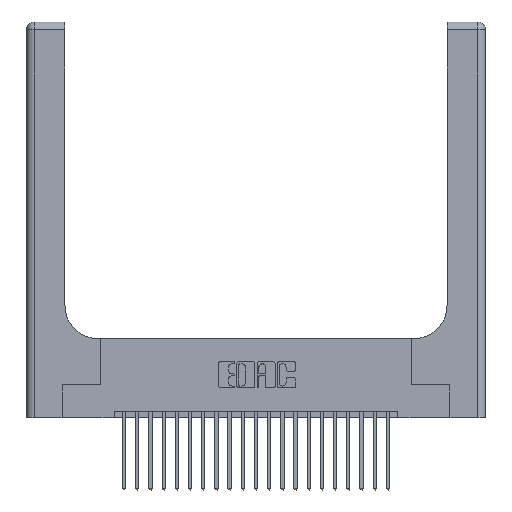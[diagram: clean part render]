
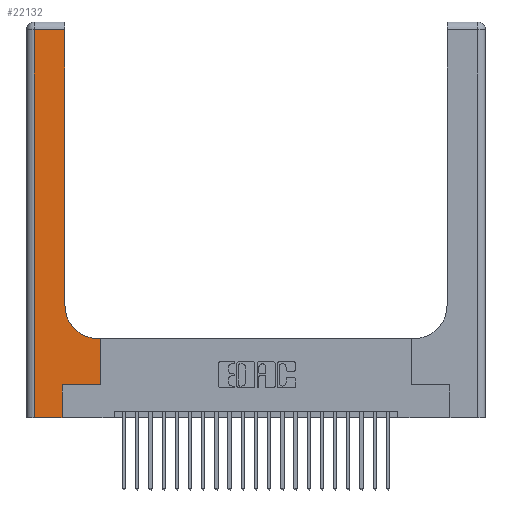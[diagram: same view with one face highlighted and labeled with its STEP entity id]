
A CAD part, top view. The second image highlights one B-rep face of the part: STEP entity #22132.
In plain terms, the highlighted planar face has unit normal (0, 0, 1).
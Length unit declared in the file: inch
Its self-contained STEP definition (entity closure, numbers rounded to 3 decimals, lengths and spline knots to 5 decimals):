
#15 = ORIENTED_EDGE ( 'NONE', *, *, #10885, .T. ) ;
#151 = VECTOR ( 'NONE', #19721, 39.37008 ) ;
#191 = VERTEX_POINT ( 'NONE', #14990 ) ;
#304 = ORIENTED_EDGE ( 'NONE', *, *, #4779, .T. ) ;
#628 = EDGE_CURVE ( 'NONE', #14026, #11535, #16744, .T. ) ;
#1269 = LINE ( 'NONE', #4823, #3941 ) ;
#1821 = ORIENTED_EDGE ( 'NONE', *, *, #12774, .T. ) ;
#1861 = LINE ( 'NONE', #20226, #16355 ) ;
#2771 = VERTEX_POINT ( 'NONE', #4696 ) ;
#2961 = DIRECTION ( 'NONE',  ( 0., -1., 0. ) ) ;
#3645 = CARTESIAN_POINT ( 'NONE',  ( 0.5415, 0.85, 0.37 ) ) ;
#3941 = VECTOR ( 'NONE', #14486, 39.37008 ) ;
#4376 = VECTOR ( 'NONE', #17408, 39.37008 ) ;
#4696 = CARTESIAN_POINT ( 'NONE',  ( 0.5415, 0.6, 0.37 ) ) ;
#4779 = EDGE_CURVE ( 'NONE', #11535, #2771, #18052, .T. ) ;
#4823 = CARTESIAN_POINT ( 'NONE',  ( 0.269, 0.25, 0.37 ) ) ;
#5253 = ORIENTED_EDGE ( 'NONE', *, *, #23260, .T. ) ;
#5434 = ORIENTED_EDGE ( 'NONE', *, *, #628, .T. ) ;
#6250 = ORIENTED_EDGE ( 'NONE', *, *, #9044, .T. ) ;
#6401 = VECTOR ( 'NONE', #20371, 39.37008 ) ;
#6439 = CARTESIAN_POINT ( 'NONE',  ( 0.269, 0.25, 0.37 ) ) ;
#6576 = CARTESIAN_POINT ( 'NONE',  ( 0.06, 2.94, 0.37 ) ) ;
#6899 = DIRECTION ( 'NONE',  ( -1., 0., 0. ) ) ;
#7029 = LINE ( 'NONE', #17320, #4376 ) ;
#7435 = EDGE_CURVE ( 'NONE', #23414, #21088, #10299, .T. ) ;
#8166 = CARTESIAN_POINT ( 'NONE',  ( 0., 3., 0.37 ) ) ;
#8260 = DIRECTION ( 'NONE',  ( -1., 0., 0. ) ) ;
#9044 = EDGE_CURVE ( 'NONE', #14669, #16387, #12584, .T. ) ;
#9825 = LINE ( 'NONE', #14410, #12785 ) ;
#9915 = DIRECTION ( 'NONE',  ( 0., 0., -1. ) ) ;
#10299 = LINE ( 'NONE', #21711, #151 ) ;
#10885 = EDGE_CURVE ( 'NONE', #21088, #16942, #9825, .T. ) ;
#11535 = VERTEX_POINT ( 'NONE', #16515 ) ;
#11664 = CARTESIAN_POINT ( 'NONE',  ( 0.269, 0., 0.37 ) ) ;
#11736 = ORIENTED_EDGE ( 'NONE', *, *, #7435, .T. ) ;
#11746 = CARTESIAN_POINT ( 'NONE',  ( 0.2915, 0.85, 0.37 ) ) ;
#12584 = LINE ( 'NONE', #16120, #16401 ) ;
#12774 = EDGE_CURVE ( 'NONE', #16387, #14026, #1269, .T. ) ;
#12785 = VECTOR ( 'NONE', #6899, 39.37008 ) ;
#13027 = EDGE_CURVE ( 'NONE', #16942, #191, #1861, .T. ) ;
#13786 = ORIENTED_EDGE ( 'NONE', *, *, #13027, .T. ) ;
#14026 = VERTEX_POINT ( 'NONE', #23121 ) ;
#14341 = CIRCLE ( 'NONE', #19201, 0.25 ) ;
#14410 = CARTESIAN_POINT ( 'NONE',  ( 0., 2.94, 0.37 ) ) ;
#14486 = DIRECTION ( 'NONE',  ( 1., 0., 0. ) ) ;
#14669 = VERTEX_POINT ( 'NONE', #11664 ) ;
#14990 = CARTESIAN_POINT ( 'NONE',  ( 0.06, 0., 0.37 ) ) ;
#15864 = CARTESIAN_POINT ( 'NONE',  ( 0.2915, 2.94, 0.37 ) ) ;
#16120 = CARTESIAN_POINT ( 'NONE',  ( 0.269, 0., 0.37 ) ) ;
#16189 = EDGE_CURVE ( 'NONE', #191, #14669, #7029, .T. ) ;
#16355 = VECTOR ( 'NONE', #2961, 39.37008 ) ;
#16387 = VERTEX_POINT ( 'NONE', #6439 ) ;
#16401 = VECTOR ( 'NONE', #22045, 39.37008 ) ;
#16515 = CARTESIAN_POINT ( 'NONE',  ( 0.5585, 0.6, 0.37 ) ) ;
#16744 = LINE ( 'NONE', #22371, #6401 ) ;
#16942 = VERTEX_POINT ( 'NONE', #6576 ) ;
#17018 = DIRECTION ( 'NONE',  ( 0., 0., -1. ) ) ;
#17320 = CARTESIAN_POINT ( 'NONE',  ( 0., 0., 0.37 ) ) ;
#17408 = DIRECTION ( 'NONE',  ( 1., 0., 0. ) ) ;
#18052 = LINE ( 'NONE', #23661, #20083 ) ;
#19201 = AXIS2_PLACEMENT_3D ( 'NONE', #3645, #17018, #24378 ) ;
#19721 = DIRECTION ( 'NONE',  ( 0., 1., 0. ) ) ;
#20083 = VECTOR ( 'NONE', #24305, 39.37008 ) ;
#20226 = CARTESIAN_POINT ( 'NONE',  ( 0.06, 3., 0.37 ) ) ;
#20371 = DIRECTION ( 'NONE',  ( 0., 1., 0. ) ) ;
#20582 = EDGE_LOOP ( 'NONE', ( #11736, #15, #13786, #22025, #6250, #1821, #5434, #304, #5253 ) ) ;
#21087 = AXIS2_PLACEMENT_3D ( 'NONE', #8166, #9915, #8260 ) ;
#21088 = VERTEX_POINT ( 'NONE', #15864 ) ;
#21191 = PLANE ( 'NONE',  #21087 ) ;
#21711 = CARTESIAN_POINT ( 'NONE',  ( 0.2915, 3., 0.37 ) ) ;
#22025 = ORIENTED_EDGE ( 'NONE', *, *, #16189, .T. ) ;
#22045 = DIRECTION ( 'NONE',  ( 0., 1., 0. ) ) ;
#22132 = ADVANCED_FACE ( 'NONE', ( #22356 ), #21191, .F. ) ;
#22356 = FACE_OUTER_BOUND ( 'NONE', #20582, .T. ) ;
#22371 = CARTESIAN_POINT ( 'NONE',  ( 0.5585, 0.25, 0.37 ) ) ;
#23121 = CARTESIAN_POINT ( 'NONE',  ( 0.5585, 0.25, 0.37 ) ) ;
#23260 = EDGE_CURVE ( 'NONE', #2771, #23414, #14341, .T. ) ;
#23414 = VERTEX_POINT ( 'NONE', #11746 ) ;
#23661 = CARTESIAN_POINT ( 'NONE',  ( 0.2915, 0.6, 0.37 ) ) ;
#24305 = DIRECTION ( 'NONE',  ( -1., 0., 0. ) ) ;
#24378 = DIRECTION ( 'NONE',  ( 1., 0., 0. ) ) ;
